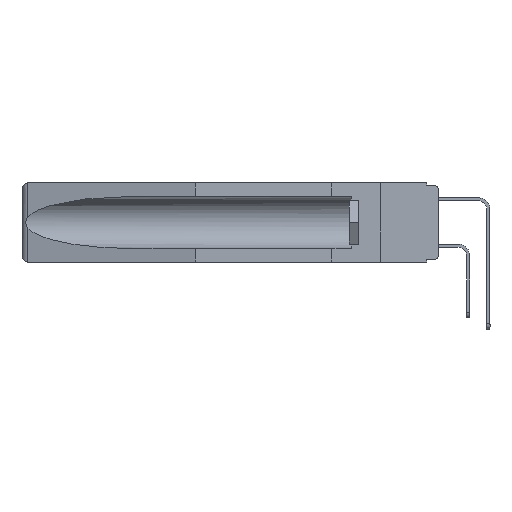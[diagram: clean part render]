
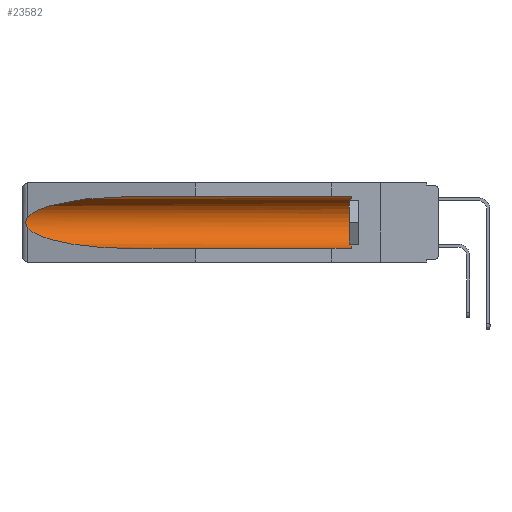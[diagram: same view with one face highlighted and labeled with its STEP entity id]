
A CAD part, left-side view. The second image highlights one B-rep face of the part: STEP entity #23582.
In plain terms, the highlighted cylindrical face has radius 2.857 mm (diameter 5.715 mm), a partial arc.
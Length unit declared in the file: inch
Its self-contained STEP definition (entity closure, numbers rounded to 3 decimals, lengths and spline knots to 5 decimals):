
#176 = CARTESIAN_POINT ( 'NONE',  ( 0.155, -0.30754, -0.059 ) ) ;
#383 =( BOUNDED_CURVE ( )  B_SPLINE_CURVE ( 3, ( #22316, #18494, #24660, #17915 ),
 .UNSPECIFIED., .F., .F. ) 
 B_SPLINE_CURVE_WITH_KNOTS ( ( 4, 4 ),
 ( 4.71239, 6.08839 ),
 .UNSPECIFIED. ) 
 CURVE ( )  GEOMETRIC_REPRESENTATION_ITEM ( )  RATIONAL_B_SPLINE_CURVE ( ( 1., 0.848, 0.848, 1. ) ) 
 REPRESENTATION_ITEM ( '' )  );
#1405 = VERTEX_POINT ( 'NONE', #15836 ) ;
#1415 = CARTESIAN_POINT ( 'NONE',  ( 0.2675, 1.53308, -0.16763 ) ) ;
#1612 = EDGE_CURVE ( 'NONE', #4918, #17978, #16750, .T. ) ;
#2420 = CARTESIAN_POINT ( 'NONE',  ( 0.155, -0.30754, -0.284 ) ) ;
#2899 = VECTOR ( 'NONE', #11891, 39.37008 ) ;
#3789 = CARTESIAN_POINT ( 'NONE',  ( 0.25451, 1.48313, -0.24835 ) ) ;
#4863 = ORIENTED_EDGE ( 'NONE', *, *, #27417, .T. ) ;
#4918 = VERTEX_POINT ( 'NONE', #10060 ) ;
#5164 = EDGE_LOOP ( 'NONE', ( #24249, #8267, #4863, #16378, #24923, #12347 ) ) ;
#5228 =( BOUNDED_CURVE ( )  B_SPLINE_CURVE ( 3, ( #17332, #3789, #22012, #28175 ),
 .UNSPECIFIED., .F., .T. ) 
 B_SPLINE_CURVE_WITH_KNOTS ( ( 4, 4 ),
 ( 0.1948, 1.5708 ),
 .UNSPECIFIED. ) 
 CURVE ( )  GEOMETRIC_REPRESENTATION_ITEM ( )  RATIONAL_B_SPLINE_CURVE ( ( 1., 0.848, 0.848, 1. ) ) 
 REPRESENTATION_ITEM ( '' )  );
#5395 = CARTESIAN_POINT ( 'NONE',  ( 0.155, -0.30754, -0.1715 ) ) ;
#5692 = DIRECTION ( 'NONE',  ( 0., 1., 0. ) ) ;
#5936 = CARTESIAN_POINT ( 'NONE',  ( 0.26597, 1.52961, -0.15275 ) ) ;
#6520 = CARTESIAN_POINT ( 'NONE',  ( 0.26537, 1.52718, -0.19328 ) ) ;
#6635 = CIRCLE ( 'NONE', #11349, 0.1125 ) ;
#7791 = VERTEX_POINT ( 'NONE', #13740 ) ;
#7953 = DIRECTION ( 'NONE',  ( 0., -1., 0. ) ) ;
#8145 = CARTESIAN_POINT ( 'NONE',  ( 0.26655, 1.53094, -0.18657 ) ) ;
#8267 = ORIENTED_EDGE ( 'NONE', *, *, #1612, .T. ) ;
#8840 = CARTESIAN_POINT ( 'NONE',  ( 0.26537, 1.52718, -0.19328 ) ) ;
#9392 = EDGE_CURVE ( 'NONE', #1405, #14647, #22524, .T. ) ;
#10060 = CARTESIAN_POINT ( 'NONE',  ( 0.26537, 1.52718, -0.14972 ) ) ;
#11349 = AXIS2_PLACEMENT_3D ( 'NONE', #28092, #7953, #16947 ) ;
#11891 = DIRECTION ( 'NONE',  ( 0., 1., 0. ) ) ;
#12172 = FACE_OUTER_BOUND ( 'NONE', #5164, .T. ) ;
#12347 = ORIENTED_EDGE ( 'NONE', *, *, #14935, .T. ) ;
#12706 = CARTESIAN_POINT ( 'NONE',  ( 0.2675, 1.53308, -0.17534 ) ) ;
#13324 = EDGE_CURVE ( 'NONE', #1405, #7791, #6635, .T. ) ;
#13740 = CARTESIAN_POINT ( 'NONE',  ( 0.155, 0.126, -0.059 ) ) ;
#14647 = VERTEX_POINT ( 'NONE', #17092 ) ;
#14935 = EDGE_CURVE ( 'NONE', #7791, #28574, #22928, .T. ) ;
#15075 = CARTESIAN_POINT ( 'NONE',  ( 0.2673, 1.5327, -0.16383 ) ) ;
#15206 = DIRECTION ( 'NONE',  ( 0., 1., 0. ) ) ;
#15285 = EDGE_CURVE ( 'NONE', #28574, #4918, #383, .T. ) ;
#15836 = CARTESIAN_POINT ( 'NONE',  ( 0.155, 0.126, -0.284 ) ) ;
#16378 = ORIENTED_EDGE ( 'NONE', *, *, #9392, .F. ) ;
#16479 = CARTESIAN_POINT ( 'NONE',  ( 0.155, 1.07973, -0.059 ) ) ;
#16750 = B_SPLINE_CURVE_WITH_KNOTS ( 'NONE', 3,
 ( #22111, #5936, #19767, #15075, #1415, #12706, #17281, #8145, #23879, #6520 ),
 .UNSPECIFIED., .F., .F.,
 ( 4, 2, 2, 2, 4 ),
 ( 0., 0.00029, 0.00058, 0.00087, 0.00117 ),
 .UNSPECIFIED. ) ;
#16947 = DIRECTION ( 'NONE',  ( 0., 0., 1. ) ) ;
#17092 = CARTESIAN_POINT ( 'NONE',  ( 0.155, 1.07973, -0.284 ) ) ;
#17281 = CARTESIAN_POINT ( 'NONE',  ( 0.2673, 1.53269, -0.17917 ) ) ;
#17332 = CARTESIAN_POINT ( 'NONE',  ( 0.26537, 1.52718, -0.19328 ) ) ;
#17915 = CARTESIAN_POINT ( 'NONE',  ( 0.26537, 1.52718, -0.14972 ) ) ;
#17978 = VERTEX_POINT ( 'NONE', #8840 ) ;
#18494 = CARTESIAN_POINT ( 'NONE',  ( 0.21114, 1.30732, -0.059 ) ) ;
#19767 = CARTESIAN_POINT ( 'NONE',  ( 0.26654, 1.53092, -0.15636 ) ) ;
#20127 = AXIS2_PLACEMENT_3D ( 'NONE', #5395, #5692, #21145 ) ;
#21145 = DIRECTION ( 'NONE',  ( 0., 0., 1. ) ) ;
#21282 = CYLINDRICAL_SURFACE ( 'NONE', #20127, 0.1125 ) ;
#22012 = CARTESIAN_POINT ( 'NONE',  ( 0.21114, 1.30732, -0.284 ) ) ;
#22111 = CARTESIAN_POINT ( 'NONE',  ( 0.26537, 1.52718, -0.14972 ) ) ;
#22316 = CARTESIAN_POINT ( 'NONE',  ( 0.155, 1.07973, -0.059 ) ) ;
#22524 = LINE ( 'NONE', #2420, #28656 ) ;
#22928 = LINE ( 'NONE', #176, #2899 ) ;
#23582 = ADVANCED_FACE ( 'NONE', ( #12172 ), #21282, .F. ) ;
#23879 = CARTESIAN_POINT ( 'NONE',  ( 0.26597, 1.5296, -0.19026 ) ) ;
#24249 = ORIENTED_EDGE ( 'NONE', *, *, #15285, .T. ) ;
#24660 = CARTESIAN_POINT ( 'NONE',  ( 0.25451, 1.48313, -0.09465 ) ) ;
#24923 = ORIENTED_EDGE ( 'NONE', *, *, #13324, .T. ) ;
#27417 = EDGE_CURVE ( 'NONE', #17978, #14647, #5228, .T. ) ;
#28092 = CARTESIAN_POINT ( 'NONE',  ( 0.155, 0.126, -0.1715 ) ) ;
#28175 = CARTESIAN_POINT ( 'NONE',  ( 0.155, 1.07973, -0.284 ) ) ;
#28574 = VERTEX_POINT ( 'NONE', #16479 ) ;
#28656 = VECTOR ( 'NONE', #15206, 39.37008 ) ;
